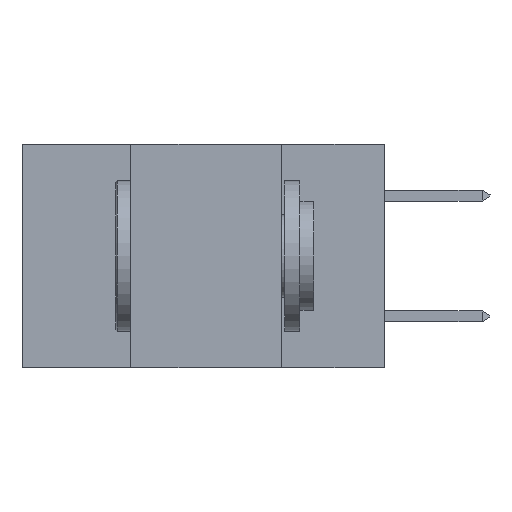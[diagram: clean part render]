
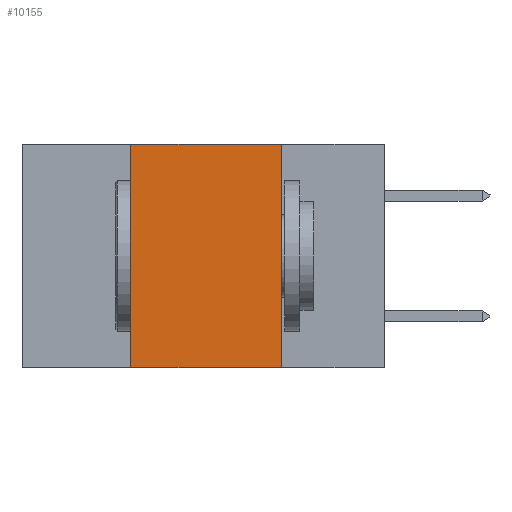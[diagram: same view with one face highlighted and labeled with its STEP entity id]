
A CAD part, left-side view. The second image highlights one B-rep face of the part: STEP entity #10155.
In plain terms, the highlighted planar face has unit normal (-1, 0, 0).
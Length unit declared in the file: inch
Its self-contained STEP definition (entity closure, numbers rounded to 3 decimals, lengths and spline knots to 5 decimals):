
#359 = VECTOR ( 'NONE', #7836, 39.37008 ) ;
#1804 = CARTESIAN_POINT ( 'NONE',  ( 0., 0.17, -0.37 ) ) ;
#3536 = EDGE_CURVE ( 'NONE', #16962, #10060, #17720, .T. ) ;
#5134 = CARTESIAN_POINT ( 'NONE',  ( 0., 0.42, 0. ) ) ;
#5868 = EDGE_LOOP ( 'NONE', ( #19310, #27652, #32362, #26071 ) ) ;
#7357 = FACE_OUTER_BOUND ( 'NONE', #5868, .T. ) ;
#7836 = DIRECTION ( 'NONE',  ( 0., 0., -1. ) ) ;
#9397 = LINE ( 'NONE', #24837, #359 ) ;
#10060 = VERTEX_POINT ( 'NONE', #1804 ) ;
#10155 = ADVANCED_FACE ( 'NONE', ( #7357 ), #35987, .F. ) ;
#11929 = VECTOR ( 'NONE', #20251, 39.37008 ) ;
#12814 = CARTESIAN_POINT ( 'NONE',  ( 0., 0.17, 0. ) ) ;
#14412 = EDGE_CURVE ( 'NONE', #16962, #16489, #39452, .T. ) ;
#15185 = CARTESIAN_POINT ( 'NONE',  ( 0., 0.42, -0.37 ) ) ;
#15536 = DIRECTION ( 'NONE',  ( 1., 0., 0. ) ) ;
#15731 = LINE ( 'NONE', #16960, #11929 ) ;
#16489 = VERTEX_POINT ( 'NONE', #23609 ) ;
#16960 = CARTESIAN_POINT ( 'NONE',  ( 0., 0.6, 0. ) ) ;
#16962 = VERTEX_POINT ( 'NONE', #15185 ) ;
#17720 = LINE ( 'NONE', #30058, #39116 ) ;
#17986 = EDGE_CURVE ( 'NONE', #16489, #25167, #15731, .T. ) ;
#19310 = ORIENTED_EDGE ( 'NONE', *, *, #39410, .F. ) ;
#20251 = DIRECTION ( 'NONE',  ( 0., -1., 0. ) ) ;
#23609 = CARTESIAN_POINT ( 'NONE',  ( 0., 0.42, 0. ) ) ;
#24837 = CARTESIAN_POINT ( 'NONE',  ( 0., 0.17, 0. ) ) ;
#25167 = VERTEX_POINT ( 'NONE', #12814 ) ;
#26071 = ORIENTED_EDGE ( 'NONE', *, *, #3536, .T. ) ;
#26332 = DIRECTION ( 'NONE',  ( 0., -1., 0. ) ) ;
#27652 = ORIENTED_EDGE ( 'NONE', *, *, #17986, .F. ) ;
#30058 = CARTESIAN_POINT ( 'NONE',  ( 0., 0.6, -0.37 ) ) ;
#31401 = VECTOR ( 'NONE', #39690, 39.37008 ) ;
#32362 = ORIENTED_EDGE ( 'NONE', *, *, #14412, .F. ) ;
#33120 = AXIS2_PLACEMENT_3D ( 'NONE', #40230, #15536, #39469 ) ;
#35987 = PLANE ( 'NONE',  #33120 ) ;
#39116 = VECTOR ( 'NONE', #26332, 39.37008 ) ;
#39410 = EDGE_CURVE ( 'NONE', #25167, #10060, #9397, .T. ) ;
#39452 = LINE ( 'NONE', #5134, #31401 ) ;
#39469 = DIRECTION ( 'NONE',  ( 0., 0., -1. ) ) ;
#39690 = DIRECTION ( 'NONE',  ( 0., 0., 1. ) ) ;
#40230 = CARTESIAN_POINT ( 'NONE',  ( 0., 0.6, 0. ) ) ;
